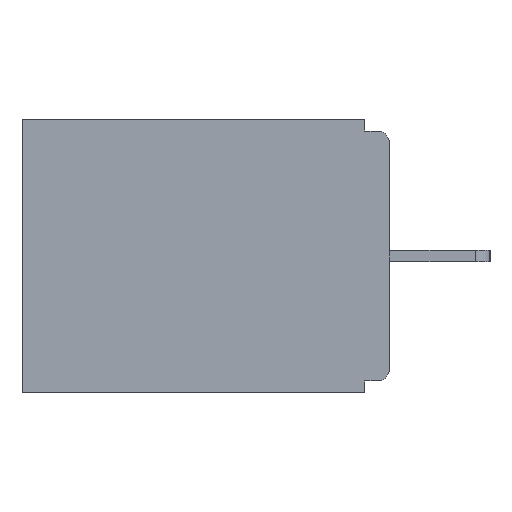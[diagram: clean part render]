
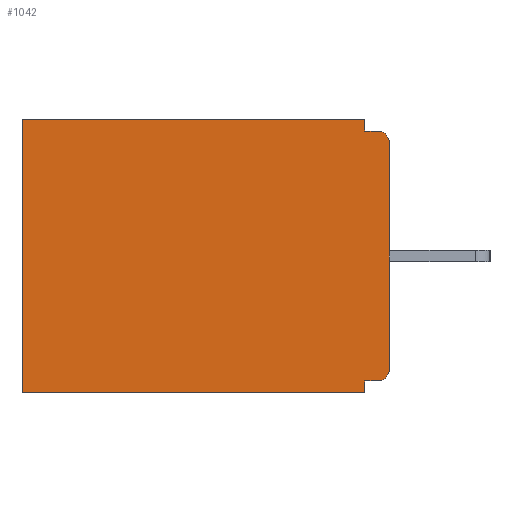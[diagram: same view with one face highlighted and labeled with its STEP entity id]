
A CAD part, left-side view. The second image highlights one B-rep face of the part: STEP entity #1042.
In plain terms, the highlighted planar face has unit normal (-1, 0, 0).
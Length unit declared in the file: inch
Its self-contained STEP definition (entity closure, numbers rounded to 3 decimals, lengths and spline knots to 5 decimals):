
#3 = LINE ( 'NONE', #22038, #4694 ) ;
#194 = CARTESIAN_POINT ( 'NONE',  ( 0.298, 0.015, -0.328 ) ) ;
#388 = CARTESIAN_POINT ( 'NONE',  ( 0.298, 0.015, -0.015 ) ) ;
#576 = LINE ( 'NONE', #13744, #10249 ) ;
#616 = ORIENTED_EDGE ( 'NONE', *, *, #12086, .F. ) ;
#1042 = ADVANCED_FACE ( 'NONE', ( #23030 ), #7293, .F. ) ;
#1046 = DIRECTION ( 'NONE',  ( 0., -1., 0. ) ) ;
#1272 = EDGE_CURVE ( 'NONE', #16108, #2517, #14386, .T. ) ;
#1276 = VERTEX_POINT ( 'NONE', #388 ) ;
#1403 = CARTESIAN_POINT ( 'NONE',  ( 0.298, 0., -0.03 ) ) ;
#2383 = VECTOR ( 'NONE', #14912, 39.37008 ) ;
#2517 = VERTEX_POINT ( 'NONE', #22025 ) ;
#2852 = DIRECTION ( 'NONE',  ( 0., 0., -1. ) ) ;
#2943 = AXIS2_PLACEMENT_3D ( 'NONE', #21328, #21166, #21026 ) ;
#3121 = CARTESIAN_POINT ( 'NONE',  ( 0.298, 0.031, -0.343 ) ) ;
#3400 = VERTEX_POINT ( 'NONE', #22785 ) ;
#3649 = VERTEX_POINT ( 'NONE', #23792 ) ;
#3948 = EDGE_CURVE ( 'NONE', #16108, #1276, #19458, .T. ) ;
#4397 = DIRECTION ( 'NONE',  ( 0., 1., 0. ) ) ;
#4694 = VECTOR ( 'NONE', #23752, 39.37008 ) ;
#5052 = CARTESIAN_POINT ( 'NONE',  ( 0.298, 0.46, 0. ) ) ;
#5120 = ORIENTED_EDGE ( 'NONE', *, *, #13636, .F. ) ;
#5302 = LINE ( 'NONE', #3121, #23549 ) ;
#5360 = VERTEX_POINT ( 'NONE', #13261 ) ;
#5518 = DIRECTION ( 'NONE',  ( 0., 1., 0. ) ) ;
#6571 = ORIENTED_EDGE ( 'NONE', *, *, #1272, .F. ) ;
#6705 = VECTOR ( 'NONE', #1046, 39.37008 ) ;
#7183 = VERTEX_POINT ( 'NONE', #20280 ) ;
#7222 = CARTESIAN_POINT ( 'NONE',  ( 0.298, 0.031, 0. ) ) ;
#7230 = ORIENTED_EDGE ( 'NONE', *, *, #12865, .F. ) ;
#7293 = PLANE ( 'NONE',  #14375 ) ;
#7552 = ORIENTED_EDGE ( 'NONE', *, *, #11477, .F. ) ;
#7891 = VECTOR ( 'NONE', #5518, 39.37008 ) ;
#8093 = DIRECTION ( 'NONE',  ( 0., 0., -1. ) ) ;
#8809 = ORIENTED_EDGE ( 'NONE', *, *, #8940, .F. ) ;
#8940 = EDGE_CURVE ( 'NONE', #15670, #3400, #16253, .T. ) ;
#8966 = CARTESIAN_POINT ( 'NONE',  ( 0.298, 0., -0.343 ) ) ;
#9064 = LINE ( 'NONE', #10330, #6705 ) ;
#9155 = CARTESIAN_POINT ( 'NONE',  ( 0.298, 0.46, 0. ) ) ;
#9288 = EDGE_CURVE ( 'NONE', #21736, #2517, #9488, .T. ) ;
#9406 = VECTOR ( 'NONE', #8093, 39.37008 ) ;
#9425 = LINE ( 'NONE', #9155, #2383 ) ;
#9488 = CIRCLE ( 'NONE', #18591, 0.015 ) ;
#9711 = CARTESIAN_POINT ( 'NONE',  ( 0.298, 0.015, -0.313 ) ) ;
#10249 = VECTOR ( 'NONE', #4397, 39.37008 ) ;
#10330 = CARTESIAN_POINT ( 'NONE',  ( 0.298, 0., -0.015 ) ) ;
#10985 = DIRECTION ( 'NONE',  ( 1., 0., 0. ) ) ;
#11175 = ORIENTED_EDGE ( 'NONE', *, *, #18771, .T. ) ;
#11239 = VECTOR ( 'NONE', #2852, 39.37008 ) ;
#11477 = EDGE_CURVE ( 'NONE', #3400, #1276, #9064, .T. ) ;
#12086 = EDGE_CURVE ( 'NONE', #3649, #7183, #5302, .T. ) ;
#12865 = EDGE_CURVE ( 'NONE', #21736, #3649, #576, .T. ) ;
#13261 = CARTESIAN_POINT ( 'NONE',  ( 0.298, 0.46, -0.343 ) ) ;
#13636 = EDGE_CURVE ( 'NONE', #7183, #5360, #16701, .T. ) ;
#13733 = CARTESIAN_POINT ( 'NONE',  ( 0.298, 0., 0. ) ) ;
#13744 = CARTESIAN_POINT ( 'NONE',  ( 0.298, 0., -0.328 ) ) ;
#14284 = DIRECTION ( 'NONE',  ( 0., 0., -1. ) ) ;
#14375 = AXIS2_PLACEMENT_3D ( 'NONE', #24060, #10985, #16579 ) ;
#14386 = LINE ( 'NONE', #13733, #9406 ) ;
#14833 = ORIENTED_EDGE ( 'NONE', *, *, #3948, .T. ) ;
#14912 = DIRECTION ( 'NONE',  ( 0., 0., -1. ) ) ;
#15157 = EDGE_CURVE ( 'NONE', #15670, #15919, #3, .T. ) ;
#15670 = VERTEX_POINT ( 'NONE', #7222 ) ;
#15789 = ORIENTED_EDGE ( 'NONE', *, *, #9288, .T. ) ;
#15919 = VERTEX_POINT ( 'NONE', #5052 ) ;
#16056 = ORIENTED_EDGE ( 'NONE', *, *, #15157, .T. ) ;
#16108 = VERTEX_POINT ( 'NONE', #1403 ) ;
#16253 = LINE ( 'NONE', #19701, #11239 ) ;
#16579 = DIRECTION ( 'NONE',  ( 0., 0., -1. ) ) ;
#16701 = LINE ( 'NONE', #8966, #7891 ) ;
#18591 = AXIS2_PLACEMENT_3D ( 'NONE', #9711, #22996, #22840 ) ;
#18771 = EDGE_CURVE ( 'NONE', #15919, #5360, #9425, .T. ) ;
#19458 = CIRCLE ( 'NONE', #2943, 0.015 ) ;
#19701 = CARTESIAN_POINT ( 'NONE',  ( 0.298, 0.031, -0.343 ) ) ;
#20280 = CARTESIAN_POINT ( 'NONE',  ( 0.298, 0.031, -0.343 ) ) ;
#20809 = EDGE_LOOP ( 'NONE', ( #14833, #7552, #8809, #16056, #11175, #5120, #616, #7230, #15789, #6571 ) ) ;
#21026 = DIRECTION ( 'NONE',  ( 0., 0., -1. ) ) ;
#21166 = DIRECTION ( 'NONE',  ( -1., 0., 0. ) ) ;
#21328 = CARTESIAN_POINT ( 'NONE',  ( 0.298, 0.015, -0.03 ) ) ;
#21736 = VERTEX_POINT ( 'NONE', #194 ) ;
#22025 = CARTESIAN_POINT ( 'NONE',  ( 0.298, 0., -0.313 ) ) ;
#22038 = CARTESIAN_POINT ( 'NONE',  ( 0.298, 0., 0. ) ) ;
#22785 = CARTESIAN_POINT ( 'NONE',  ( 0.298, 0.031, -0.015 ) ) ;
#22840 = DIRECTION ( 'NONE',  ( 0., 0., -1. ) ) ;
#22996 = DIRECTION ( 'NONE',  ( -1., 0., 0. ) ) ;
#23030 = FACE_OUTER_BOUND ( 'NONE', #20809, .T. ) ;
#23549 = VECTOR ( 'NONE', #14284, 39.37008 ) ;
#23752 = DIRECTION ( 'NONE',  ( 0., 1., 0. ) ) ;
#23792 = CARTESIAN_POINT ( 'NONE',  ( 0.298, 0.031, -0.328 ) ) ;
#24060 = CARTESIAN_POINT ( 'NONE',  ( 0.298, 0., 0. ) ) ;
